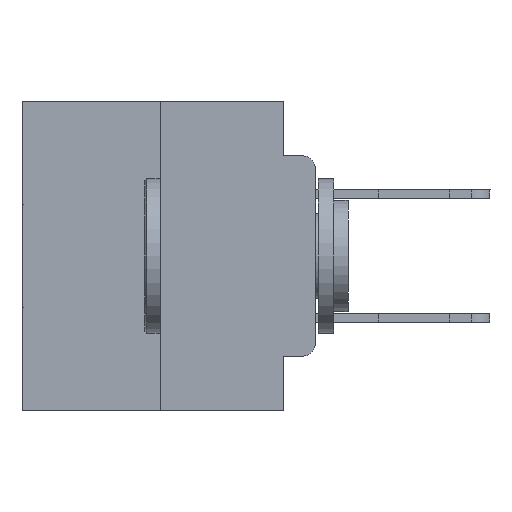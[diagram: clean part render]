
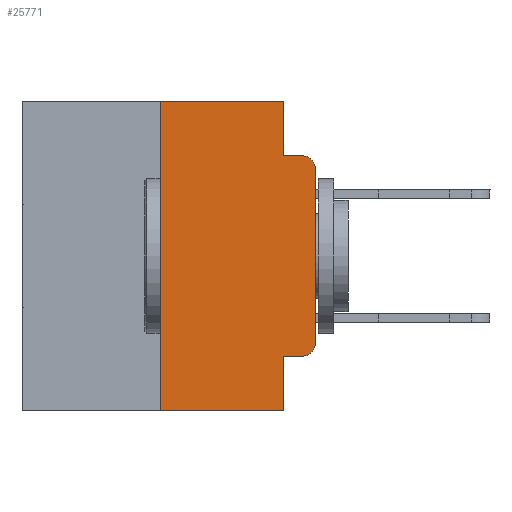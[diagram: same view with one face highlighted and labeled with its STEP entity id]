
A CAD part, left-side view. The second image highlights one B-rep face of the part: STEP entity #25771.
In plain terms, the highlighted planar face has unit normal (-1, 0, 0).
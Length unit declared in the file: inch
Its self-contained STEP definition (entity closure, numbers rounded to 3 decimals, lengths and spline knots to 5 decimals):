
#88 = VERTEX_POINT ( 'NONE', #18882 ) ;
#171 = VECTOR ( 'NONE', #27180, 39.37008 ) ;
#891 = LINE ( 'NONE', #10608, #171 ) ;
#1218 = FACE_OUTER_BOUND ( 'NONE', #29346, .T. ) ;
#1285 = LINE ( 'NONE', #14840, #29171 ) ;
#1331 = LINE ( 'NONE', #5843, #24911 ) ;
#1979 = CARTESIAN_POINT ( 'NONE',  ( 0., 0.051, -0.4115 ) ) ;
#2276 = EDGE_CURVE ( 'NONE', #7803, #20170, #11973, .T. ) ;
#2304 = LINE ( 'NONE', #27952, #25486 ) ;
#2386 = CARTESIAN_POINT ( 'NONE',  ( 0., 0., -0.3915 ) ) ;
#2489 = CARTESIAN_POINT ( 'NONE',  ( 0., 0.051, 0. ) ) ;
#2849 = PLANE ( 'NONE',  #13379 ) ;
#4840 = ORIENTED_EDGE ( 'NONE', *, *, #25158, .F. ) ;
#5373 = CARTESIAN_POINT ( 'NONE',  ( 0., 0.473, 0. ) ) ;
#5547 = ORIENTED_EDGE ( 'NONE', *, *, #24991, .F. ) ;
#5647 = DIRECTION ( 'NONE',  ( 0., -1., 0. ) ) ;
#5843 = CARTESIAN_POINT ( 'NONE',  ( 0., 0.25, 0. ) ) ;
#5944 = VECTOR ( 'NONE', #6686, 39.37008 ) ;
#6302 = LINE ( 'NONE', #21315, #18923 ) ;
#6427 = EDGE_CURVE ( 'NONE', #20369, #28973, #8075, .T. ) ;
#6476 = DIRECTION ( 'NONE',  ( 0., -1., 0. ) ) ;
#6579 = CARTESIAN_POINT ( 'NONE',  ( 0., 0.051, -0.4115 ) ) ;
#6686 = DIRECTION ( 'NONE',  ( 0., 0., 1. ) ) ;
#6926 = VERTEX_POINT ( 'NONE', #15348 ) ;
#7445 = ORIENTED_EDGE ( 'NONE', *, *, #14310, .F. ) ;
#7803 = VERTEX_POINT ( 'NONE', #15402 ) ;
#8075 = LINE ( 'NONE', #6579, #17795 ) ;
#8437 = DIRECTION ( 'NONE',  ( 0., -1., 0. ) ) ;
#8871 = ORIENTED_EDGE ( 'NONE', *, *, #6427, .T. ) ;
#9142 = ORIENTED_EDGE ( 'NONE', *, *, #19732, .T. ) ;
#9310 = DIRECTION ( 'NONE',  ( 0., 0., -1. ) ) ;
#9784 = ORIENTED_EDGE ( 'NONE', *, *, #18148, .T. ) ;
#10385 = AXIS2_PLACEMENT_3D ( 'NONE', #13445, #11619, #19951 ) ;
#10608 = CARTESIAN_POINT ( 'NONE',  ( 0., 0.051, 0. ) ) ;
#11619 = DIRECTION ( 'NONE',  ( -1., 0., 0. ) ) ;
#11971 = DIRECTION ( 'NONE',  ( 1., 0., 0. ) ) ;
#11973 = LINE ( 'NONE', #24316, #23538 ) ;
#12112 = LINE ( 'NONE', #20529, #5944 ) ;
#12534 = DIRECTION ( 'NONE',  ( 0., -1., 0. ) ) ;
#13379 = AXIS2_PLACEMENT_3D ( 'NONE', #5373, #11971, #19218 ) ;
#13445 = CARTESIAN_POINT ( 'NONE',  ( 0., 0.02, -0.3915 ) ) ;
#13653 = EDGE_CURVE ( 'NONE', #88, #6926, #23701, .T. ) ;
#13776 = VERTEX_POINT ( 'NONE', #2489 ) ;
#14310 = EDGE_CURVE ( 'NONE', #20369, #20170, #2304, .T. ) ;
#14840 = CARTESIAN_POINT ( 'NONE',  ( 0., 0.473, 0. ) ) ;
#15348 = CARTESIAN_POINT ( 'NONE',  ( 0., 0.02, -0.0885 ) ) ;
#15402 = CARTESIAN_POINT ( 'NONE',  ( 0., 0.25, -0.5 ) ) ;
#16006 = VERTEX_POINT ( 'NONE', #16672 ) ;
#16047 = DIRECTION ( 'NONE',  ( -1., 0., 0. ) ) ;
#16672 = CARTESIAN_POINT ( 'NONE',  ( 0., 0.25, 0. ) ) ;
#17795 = VECTOR ( 'NONE', #6476, 39.37008 ) ;
#18148 = EDGE_CURVE ( 'NONE', #28973, #26270, #26314, .T. ) ;
#18882 = CARTESIAN_POINT ( 'NONE',  ( 0., 0., -0.1085 ) ) ;
#18923 = VECTOR ( 'NONE', #5647, 39.37008 ) ;
#19218 = DIRECTION ( 'NONE',  ( 0., 0., -1. ) ) ;
#19317 = CARTESIAN_POINT ( 'NONE',  ( 0., 0.051, -0.0885 ) ) ;
#19732 = EDGE_CURVE ( 'NONE', #26270, #88, #12112, .T. ) ;
#19951 = DIRECTION ( 'NONE',  ( 0., 0., -1. ) ) ;
#20131 = EDGE_CURVE ( 'NONE', #25895, #6926, #6302, .T. ) ;
#20170 = VERTEX_POINT ( 'NONE', #28999 ) ;
#20369 = VERTEX_POINT ( 'NONE', #1979 ) ;
#20529 = CARTESIAN_POINT ( 'NONE',  ( 0., 0., 0. ) ) ;
#21315 = CARTESIAN_POINT ( 'NONE',  ( 0., 0.051, -0.0885 ) ) ;
#22021 = DIRECTION ( 'NONE',  ( 0., 0., 1. ) ) ;
#22276 = ORIENTED_EDGE ( 'NONE', *, *, #20131, .F. ) ;
#23538 = VECTOR ( 'NONE', #8437, 39.37008 ) ;
#23701 = CIRCLE ( 'NONE', #26385, 0.02 ) ;
#24316 = CARTESIAN_POINT ( 'NONE',  ( 0., 0.473, -0.5 ) ) ;
#24483 = ORIENTED_EDGE ( 'NONE', *, *, #28057, .F. ) ;
#24911 = VECTOR ( 'NONE', #22021, 39.37008 ) ;
#24991 = EDGE_CURVE ( 'NONE', #16006, #13776, #1285, .T. ) ;
#25158 = EDGE_CURVE ( 'NONE', #13776, #25895, #891, .T. ) ;
#25486 = VECTOR ( 'NONE', #27859, 39.37008 ) ;
#25771 = ADVANCED_FACE ( 'NONE', ( #1218 ), #2849, .F. ) ;
#25895 = VERTEX_POINT ( 'NONE', #19317 ) ;
#26270 = VERTEX_POINT ( 'NONE', #2386 ) ;
#26314 = CIRCLE ( 'NONE', #10385, 0.02 ) ;
#26385 = AXIS2_PLACEMENT_3D ( 'NONE', #27598, #16047, #9310 ) ;
#27144 = ORIENTED_EDGE ( 'NONE', *, *, #13653, .T. ) ;
#27180 = DIRECTION ( 'NONE',  ( 0., 0., -1. ) ) ;
#27598 = CARTESIAN_POINT ( 'NONE',  ( 0., 0.02, -0.1085 ) ) ;
#27666 = ORIENTED_EDGE ( 'NONE', *, *, #2276, .T. ) ;
#27733 = CARTESIAN_POINT ( 'NONE',  ( 0., 0.02, -0.4115 ) ) ;
#27859 = DIRECTION ( 'NONE',  ( 0., 0., -1. ) ) ;
#27952 = CARTESIAN_POINT ( 'NONE',  ( 0., 0.051, 0. ) ) ;
#28057 = EDGE_CURVE ( 'NONE', #7803, #16006, #1331, .T. ) ;
#28973 = VERTEX_POINT ( 'NONE', #27733 ) ;
#28999 = CARTESIAN_POINT ( 'NONE',  ( 0., 0.051, -0.5 ) ) ;
#29171 = VECTOR ( 'NONE', #12534, 39.37008 ) ;
#29346 = EDGE_LOOP ( 'NONE', ( #9142, #27144, #22276, #4840, #5547, #24483, #27666, #7445, #8871, #9784 ) ) ;
